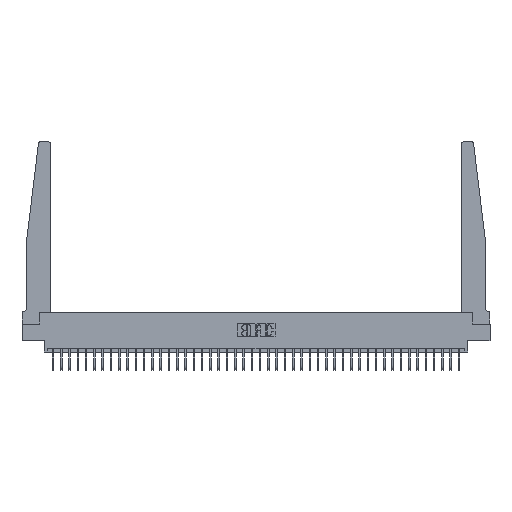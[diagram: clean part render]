
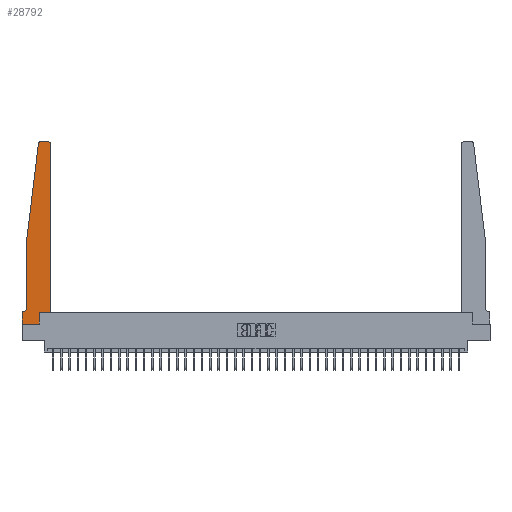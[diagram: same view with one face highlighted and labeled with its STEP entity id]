
A CAD part, top view. The second image highlights one B-rep face of the part: STEP entity #28792.
In plain terms, the highlighted planar face has unit normal (0, 0, 1).
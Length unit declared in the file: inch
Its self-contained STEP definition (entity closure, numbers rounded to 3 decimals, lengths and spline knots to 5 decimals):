
#571 = ORIENTED_EDGE ( 'NONE', *, *, #15700, .T. ) ;
#1245 = DIRECTION ( 'NONE',  ( 1., 0., 0. ) ) ;
#1705 = CARTESIAN_POINT ( 'NONE',  ( 0.24675, 2.72367, 0.37 ) ) ;
#2019 = VECTOR ( 'NONE', #2126, 39.37008 ) ;
#2027 = DIRECTION ( 'NONE',  ( 1., 0., 0. ) ) ;
#2035 = DIRECTION ( 'NONE',  ( 1., 0., 0. ) ) ;
#2126 = DIRECTION ( 'NONE',  ( 0., -1., 0. ) ) ;
#2593 = LINE ( 'NONE', #29827, #13180 ) ;
#2992 = ORIENTED_EDGE ( 'NONE', *, *, #32678, .T. ) ;
#3092 = EDGE_CURVE ( 'NONE', #15679, #12207, #7138, .T. ) ;
#3511 = LINE ( 'NONE', #12138, #34996 ) ;
#3738 = LINE ( 'NONE', #31126, #10975 ) ;
#3919 = ORIENTED_EDGE ( 'NONE', *, *, #15305, .T. ) ;
#4393 = ORIENTED_EDGE ( 'NONE', *, *, #11381, .T. ) ;
#4675 = EDGE_CURVE ( 'NONE', #8901, #10386, #10391, .T. ) ;
#5424 = LINE ( 'NONE', #5776, #31982 ) ;
#5776 = CARTESIAN_POINT ( 'NONE',  ( 0.2605, 0.18, 0.37 ) ) ;
#6005 = VERTEX_POINT ( 'NONE', #11278 ) ;
#6153 = DIRECTION ( 'NONE',  ( 1., 0., 0. ) ) ;
#6647 = VERTEX_POINT ( 'NONE', #20359 ) ;
#7138 = LINE ( 'NONE', #10182, #21413 ) ;
#7317 = VERTEX_POINT ( 'NONE', #10060 ) ;
#7425 = DIRECTION ( 'NONE',  ( -0.122, -0.992, 0. ) ) ;
#7462 = EDGE_LOOP ( 'NONE', ( #3919, #12809, #15462, #24214, #15059, #29548, #571, #24437, #4393, #7683, #2992, #22146 ) ) ;
#7487 = CARTESIAN_POINT ( 'NONE',  ( 0., 0.1875, 0.37 ) ) ;
#7683 = ORIENTED_EDGE ( 'NONE', *, *, #12840, .T. ) ;
#7944 = PLANE ( 'NONE',  #14889 ) ;
#8051 = CARTESIAN_POINT ( 'NONE',  ( 0.015, 0.2375, 0.37 ) ) ;
#8605 = VECTOR ( 'NONE', #27291, 39.37008 ) ;
#8647 = VECTOR ( 'NONE', #6153, 39.37008 ) ;
#8901 = VERTEX_POINT ( 'NONE', #21189 ) ;
#9044 = VECTOR ( 'NONE', #7425, 39.37008 ) ;
#9331 = CARTESIAN_POINT ( 'NONE',  ( 0.425, 2.72, 0.37 ) ) ;
#9503 = VERTEX_POINT ( 'NONE', #34287 ) ;
#9992 = AXIS2_PLACEMENT_3D ( 'NONE', #26941, #13500, #2035 ) ;
#10047 = CARTESIAN_POINT ( 'NONE',  ( 0.065, 1.25, 0.37 ) ) ;
#10060 = CARTESIAN_POINT ( 'NONE',  ( 0.2605, 0.18, 0.37 ) ) ;
#10182 = CARTESIAN_POINT ( 'NONE',  ( 0.065, 0.1875, 0.37 ) ) ;
#10386 = VERTEX_POINT ( 'NONE', #15610 ) ;
#10391 = LINE ( 'NONE', #10047, #2019 ) ;
#10395 = DIRECTION ( 'NONE',  ( -1., 0., 0. ) ) ;
#10975 = VECTOR ( 'NONE', #17546, 39.37008 ) ;
#11278 = CARTESIAN_POINT ( 'NONE',  ( 0.27653, 2.75, 0.37 ) ) ;
#11339 = DIRECTION ( 'NONE',  ( 0., 1., 0. ) ) ;
#11381 = EDGE_CURVE ( 'NONE', #31839, #7317, #5424, .T. ) ;
#12017 = DIRECTION ( 'NONE',  ( 0., 0., 1. ) ) ;
#12138 = CARTESIAN_POINT ( 'NONE',  ( 0., 0., 0.37 ) ) ;
#12207 = VERTEX_POINT ( 'NONE', #7487 ) ;
#12224 = CARTESIAN_POINT ( 'NONE',  ( 0.425, 0.18, 0.37 ) ) ;
#12319 = DIRECTION ( 'NONE',  ( 0., -1., 0. ) ) ;
#12809 = ORIENTED_EDGE ( 'NONE', *, *, #20336, .T. ) ;
#12840 = EDGE_CURVE ( 'NONE', #7317, #14825, #14230, .T. ) ;
#13180 = VECTOR ( 'NONE', #16584, 39.37008 ) ;
#13500 = DIRECTION ( 'NONE',  ( 0., 0., 1. ) ) ;
#14230 = LINE ( 'NONE', #33166, #8647 ) ;
#14825 = VERTEX_POINT ( 'NONE', #12224 ) ;
#14889 = AXIS2_PLACEMENT_3D ( 'NONE', #16183, #27110, #2027 ) ;
#15059 = ORIENTED_EDGE ( 'NONE', *, *, #35177, .T. ) ;
#15305 = EDGE_CURVE ( 'NONE', #6647, #6005, #3738, .T. ) ;
#15462 = ORIENTED_EDGE ( 'NONE', *, *, #29844, .T. ) ;
#15610 = CARTESIAN_POINT ( 'NONE',  ( 0.065, 0.2375, 0.37 ) ) ;
#15679 = VERTEX_POINT ( 'NONE', #17326 ) ;
#15700 = EDGE_CURVE ( 'NONE', #12207, #9503, #3511, .T. ) ;
#15945 = CIRCLE ( 'NONE', #21638, 0.03 ) ;
#16183 = CARTESIAN_POINT ( 'NONE',  ( 0., 0.1875, 0.37 ) ) ;
#16584 = DIRECTION ( 'NONE',  ( 0., 1., 0. ) ) ;
#17314 = VERTEX_POINT ( 'NONE', #1705 ) ;
#17326 = CARTESIAN_POINT ( 'NONE',  ( 0.015, 0.1875, 0.37 ) ) ;
#17546 = DIRECTION ( 'NONE',  ( -1., 0., 0. ) ) ;
#17920 = CARTESIAN_POINT ( 'NONE',  ( 0.395, 2.72, 0.37 ) ) ;
#18171 = CARTESIAN_POINT ( 'NONE',  ( 0.065, 1.25, 0.37 ) ) ;
#20336 = EDGE_CURVE ( 'NONE', #6005, #17314, #24269, .T. ) ;
#20359 = CARTESIAN_POINT ( 'NONE',  ( 0.395, 2.75, 0.37 ) ) ;
#21189 = CARTESIAN_POINT ( 'NONE',  ( 0.065, 1.25, 0.37 ) ) ;
#21413 = VECTOR ( 'NONE', #28805, 39.37008 ) ;
#21548 = FACE_OUTER_BOUND ( 'NONE', #7462, .T. ) ;
#21638 = AXIS2_PLACEMENT_3D ( 'NONE', #17920, #12017, #1245 ) ;
#22095 = LINE ( 'NONE', #32277, #8605 ) ;
#22146 = ORIENTED_EDGE ( 'NONE', *, *, #30705, .T. ) ;
#23822 = DIRECTION ( 'NONE',  ( 0., 0., -1. ) ) ;
#24214 = ORIENTED_EDGE ( 'NONE', *, *, #4675, .T. ) ;
#24269 = CIRCLE ( 'NONE', #9992, 0.03 ) ;
#24437 = ORIENTED_EDGE ( 'NONE', *, *, #34354, .T. ) ;
#25246 = CIRCLE ( 'NONE', #26382, 0.05 ) ;
#25272 = CARTESIAN_POINT ( 'NONE',  ( 0.2605, 0., 0.37 ) ) ;
#26382 = AXIS2_PLACEMENT_3D ( 'NONE', #8051, #23822, #10395 ) ;
#26941 = CARTESIAN_POINT ( 'NONE',  ( 0.27653, 2.72, 0.37 ) ) ;
#27110 = DIRECTION ( 'NONE',  ( 0., 0., 1. ) ) ;
#27291 = DIRECTION ( 'NONE',  ( 1., 0., 0. ) ) ;
#28792 = ADVANCED_FACE ( 'NONE', ( #21548 ), #7944, .T. ) ;
#28805 = DIRECTION ( 'NONE',  ( -1., 0., 0. ) ) ;
#29091 = LINE ( 'NONE', #18171, #9044 ) ;
#29548 = ORIENTED_EDGE ( 'NONE', *, *, #3092, .T. ) ;
#29827 = CARTESIAN_POINT ( 'NONE',  ( 0.425, 0.18, 0.37 ) ) ;
#29844 = EDGE_CURVE ( 'NONE', #17314, #8901, #29091, .T. ) ;
#30705 = EDGE_CURVE ( 'NONE', #32011, #6647, #15945, .T. ) ;
#31126 = CARTESIAN_POINT ( 'NONE',  ( 0.25, 2.75, 0.37 ) ) ;
#31839 = VERTEX_POINT ( 'NONE', #25272 ) ;
#31982 = VECTOR ( 'NONE', #11339, 39.37008 ) ;
#32011 = VERTEX_POINT ( 'NONE', #9331 ) ;
#32277 = CARTESIAN_POINT ( 'NONE',  ( 0., 0., 0.37 ) ) ;
#32678 = EDGE_CURVE ( 'NONE', #14825, #32011, #2593, .T. ) ;
#33166 = CARTESIAN_POINT ( 'NONE',  ( 0.425, 0.18, 0.37 ) ) ;
#34287 = CARTESIAN_POINT ( 'NONE',  ( 0., 0., 0.37 ) ) ;
#34354 = EDGE_CURVE ( 'NONE', #9503, #31839, #22095, .T. ) ;
#34996 = VECTOR ( 'NONE', #12319, 39.37008 ) ;
#35177 = EDGE_CURVE ( 'NONE', #10386, #15679, #25246, .T. ) ;
